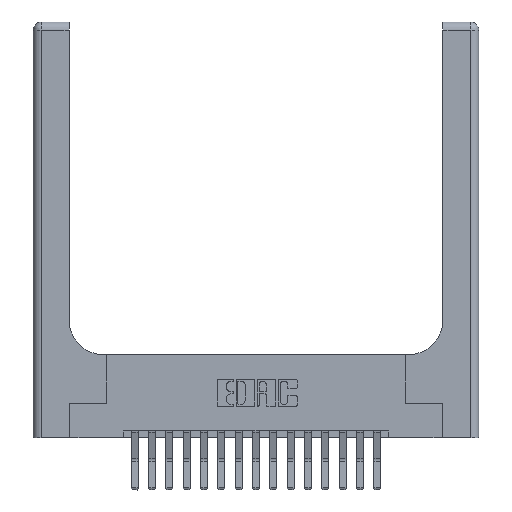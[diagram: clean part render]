
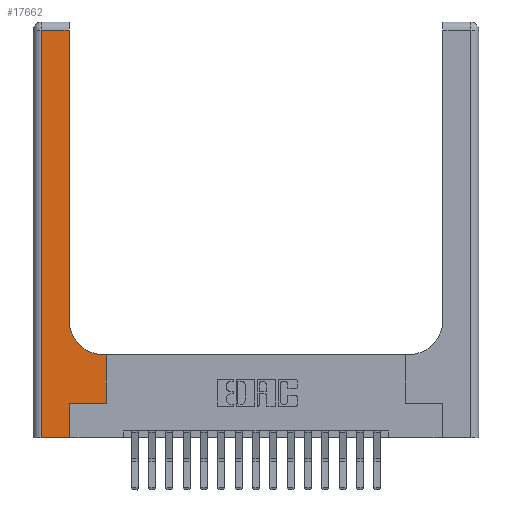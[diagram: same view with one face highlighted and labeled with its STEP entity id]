
A CAD part, top view. The second image highlights one B-rep face of the part: STEP entity #17662.
In plain terms, the highlighted planar face has unit normal (0, 0, 1).
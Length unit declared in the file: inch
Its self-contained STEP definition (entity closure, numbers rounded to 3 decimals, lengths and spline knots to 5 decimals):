
#8 = VECTOR ( 'NONE', #17674, 39.37008 ) ;
#386 = ORIENTED_EDGE ( 'NONE', *, *, #17436, .T. ) ;
#563 = VERTEX_POINT ( 'NONE', #8705 ) ;
#643 = CARTESIAN_POINT ( 'NONE',  ( 0.26, 3., 0.37 ) ) ;
#996 = EDGE_LOOP ( 'NONE', ( #16178, #14494, #15077, #15294, #11035, #386, #1359, #11989, #11748 ) ) ;
#1171 = VECTOR ( 'NONE', #12316, 39.37008 ) ;
#1359 = ORIENTED_EDGE ( 'NONE', *, *, #3702, .T. ) ;
#1713 = CARTESIAN_POINT ( 'NONE',  ( 0.528, 0.25, 0.37 ) ) ;
#2249 = CARTESIAN_POINT ( 'NONE',  ( 0., 2.94, 0.37 ) ) ;
#2287 = DIRECTION ( 'NONE',  ( -1., 0., 0. ) ) ;
#2501 = CARTESIAN_POINT ( 'NONE',  ( 0.06, 2.94, 0.37 ) ) ;
#2579 = VERTEX_POINT ( 'NONE', #5293 ) ;
#3151 = EDGE_CURVE ( 'NONE', #15712, #16825, #10191, .T. ) ;
#3190 = LINE ( 'NONE', #8117, #1171 ) ;
#3202 = DIRECTION ( 'NONE',  ( 0., -1., 0. ) ) ;
#3702 = EDGE_CURVE ( 'NONE', #12252, #3714, #12625, .T. ) ;
#3714 = VERTEX_POINT ( 'NONE', #18514 ) ;
#4405 = VECTOR ( 'NONE', #18323, 39.37008 ) ;
#4429 = DIRECTION ( 'NONE',  ( 1., 0., 0. ) ) ;
#5046 = CARTESIAN_POINT ( 'NONE',  ( 0., 3., 0.37 ) ) ;
#5155 = DIRECTION ( 'NONE',  ( 0., 1., 0. ) ) ;
#5293 = CARTESIAN_POINT ( 'NONE',  ( 0.06, 0., 0.37 ) ) ;
#5413 = DIRECTION ( 'NONE',  ( 0., 0., -1. ) ) ;
#5652 = CARTESIAN_POINT ( 'NONE',  ( 0.51, 0.6, 0.37 ) ) ;
#6354 = LINE ( 'NONE', #7419, #16292 ) ;
#7419 = CARTESIAN_POINT ( 'NONE',  ( 0.06, 3., 0.37 ) ) ;
#7828 = VERTEX_POINT ( 'NONE', #16415 ) ;
#7854 = FACE_OUTER_BOUND ( 'NONE', #996, .T. ) ;
#8117 = CARTESIAN_POINT ( 'NONE',  ( 0.26, 0.6, 0.37 ) ) ;
#8705 = CARTESIAN_POINT ( 'NONE',  ( 0.265, 0., 0.37 ) ) ;
#8824 = CARTESIAN_POINT ( 'NONE',  ( 0.265, 0., 0.37 ) ) ;
#8973 = CARTESIAN_POINT ( 'NONE',  ( 0.265, 0.25, 0.37 ) ) ;
#9161 = VECTOR ( 'NONE', #18117, 39.37008 ) ;
#9645 = VERTEX_POINT ( 'NONE', #17755 ) ;
#9996 = EDGE_CURVE ( 'NONE', #16825, #2579, #6354, .T. ) ;
#10153 = AXIS2_PLACEMENT_3D ( 'NONE', #5046, #16584, #2287 ) ;
#10191 = LINE ( 'NONE', #2249, #18104 ) ;
#10253 = EDGE_CURVE ( 'NONE', #3714, #17046, #3190, .T. ) ;
#10624 = VECTOR ( 'NONE', #5155, 39.37008 ) ;
#11035 = ORIENTED_EDGE ( 'NONE', *, *, #15157, .T. ) ;
#11157 = EDGE_CURVE ( 'NONE', #7828, #15712, #13420, .T. ) ;
#11214 = CARTESIAN_POINT ( 'NONE',  ( 0.51, 0.85, 0.37 ) ) ;
#11233 = CARTESIAN_POINT ( 'NONE',  ( 0., 0., 0.37 ) ) ;
#11748 = ORIENTED_EDGE ( 'NONE', *, *, #13611, .T. ) ;
#11989 = ORIENTED_EDGE ( 'NONE', *, *, #10253, .T. ) ;
#12252 = VERTEX_POINT ( 'NONE', #15347 ) ;
#12304 = DIRECTION ( 'NONE',  ( -1., 0., 0. ) ) ;
#12316 = DIRECTION ( 'NONE',  ( -1., 0., 0. ) ) ;
#12504 = LINE ( 'NONE', #11233, #4405 ) ;
#12625 = LINE ( 'NONE', #1713, #10624 ) ;
#12742 = AXIS2_PLACEMENT_3D ( 'NONE', #11214, #5413, #14091 ) ;
#12748 = VECTOR ( 'NONE', #4429, 39.37008 ) ;
#13420 = LINE ( 'NONE', #643, #9161 ) ;
#13611 = EDGE_CURVE ( 'NONE', #17046, #7828, #18142, .T. ) ;
#14091 = DIRECTION ( 'NONE',  ( 1., 0., 0. ) ) ;
#14494 = ORIENTED_EDGE ( 'NONE', *, *, #3151, .T. ) ;
#15077 = ORIENTED_EDGE ( 'NONE', *, *, #9996, .T. ) ;
#15157 = EDGE_CURVE ( 'NONE', #563, #9645, #18549, .T. ) ;
#15276 = LINE ( 'NONE', #8973, #12748 ) ;
#15294 = ORIENTED_EDGE ( 'NONE', *, *, #17817, .T. ) ;
#15337 = PLANE ( 'NONE',  #10153 ) ;
#15347 = CARTESIAN_POINT ( 'NONE',  ( 0.528, 0.25, 0.37 ) ) ;
#15712 = VERTEX_POINT ( 'NONE', #17536 ) ;
#16178 = ORIENTED_EDGE ( 'NONE', *, *, #11157, .T. ) ;
#16292 = VECTOR ( 'NONE', #3202, 39.37008 ) ;
#16415 = CARTESIAN_POINT ( 'NONE',  ( 0.26, 0.85, 0.37 ) ) ;
#16584 = DIRECTION ( 'NONE',  ( 0., 0., -1. ) ) ;
#16825 = VERTEX_POINT ( 'NONE', #2501 ) ;
#17046 = VERTEX_POINT ( 'NONE', #5652 ) ;
#17436 = EDGE_CURVE ( 'NONE', #9645, #12252, #15276, .T. ) ;
#17536 = CARTESIAN_POINT ( 'NONE',  ( 0.26, 2.94, 0.37 ) ) ;
#17662 = ADVANCED_FACE ( 'NONE', ( #7854 ), #15337, .F. ) ;
#17674 = DIRECTION ( 'NONE',  ( 0., 1., 0. ) ) ;
#17755 = CARTESIAN_POINT ( 'NONE',  ( 0.265, 0.25, 0.37 ) ) ;
#17817 = EDGE_CURVE ( 'NONE', #2579, #563, #12504, .T. ) ;
#18104 = VECTOR ( 'NONE', #12304, 39.37008 ) ;
#18117 = DIRECTION ( 'NONE',  ( 0., 1., 0. ) ) ;
#18142 = CIRCLE ( 'NONE', #12742, 0.25 ) ;
#18323 = DIRECTION ( 'NONE',  ( 1., 0., 0. ) ) ;
#18514 = CARTESIAN_POINT ( 'NONE',  ( 0.528, 0.6, 0.37 ) ) ;
#18549 = LINE ( 'NONE', #8824, #8 ) ;
